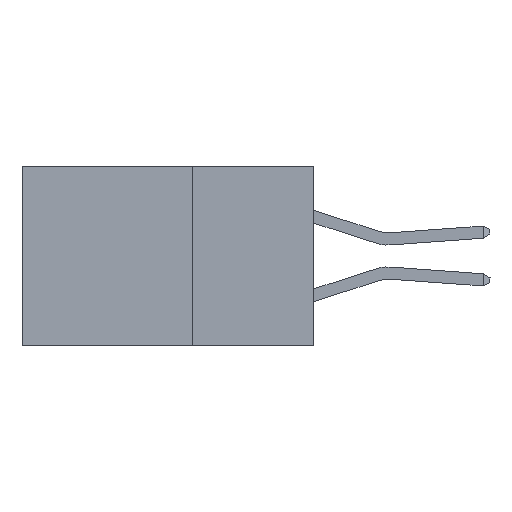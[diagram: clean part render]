
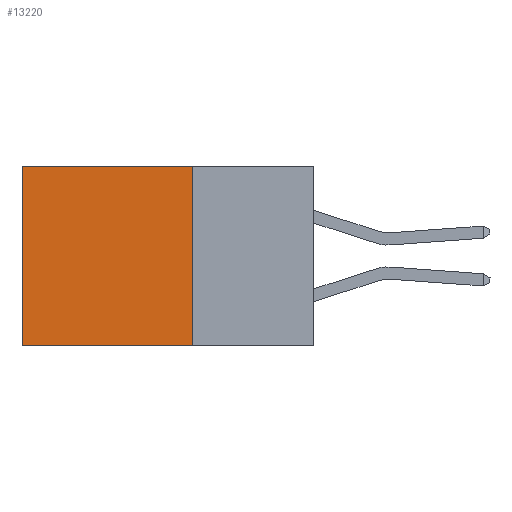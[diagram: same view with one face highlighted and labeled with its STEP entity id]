
A CAD part, left-side view. The second image highlights one B-rep face of the part: STEP entity #13220.
In plain terms, the highlighted planar face has unit normal (-1, 0, 0).
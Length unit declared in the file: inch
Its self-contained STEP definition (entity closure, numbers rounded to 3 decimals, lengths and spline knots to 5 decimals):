
#343 = VECTOR ( 'NONE', #6720, 39.37008 ) ;
#418 = CARTESIAN_POINT ( 'NONE',  ( 0.2875, 0.25, -0.37 ) ) ;
#1575 = CARTESIAN_POINT ( 'NONE',  ( 0.2875, 0.6, 0. ) ) ;
#3010 = VERTEX_POINT ( 'NONE', #418 ) ;
#3267 = PLANE ( 'NONE',  #4770 ) ;
#3728 = LINE ( 'NONE', #4398, #9536 ) ;
#3859 = VERTEX_POINT ( 'NONE', #1575 ) ;
#4029 = EDGE_CURVE ( 'NONE', #4447, #3010, #9342, .T. ) ;
#4398 = CARTESIAN_POINT ( 'NONE',  ( 0.2875, 0.25, -0.37 ) ) ;
#4447 = VERTEX_POINT ( 'NONE', #6505 ) ;
#4452 = DIRECTION ( 'NONE',  ( 0., 1., 0. ) ) ;
#4518 = DIRECTION ( 'NONE',  ( 1., 0., 0. ) ) ;
#4770 = AXIS2_PLACEMENT_3D ( 'NONE', #10228, #4518, #12395 ) ;
#4926 = ORIENTED_EDGE ( 'NONE', *, *, #6169, .T. ) ;
#5045 = FACE_OUTER_BOUND ( 'NONE', #13410, .T. ) ;
#5629 = EDGE_CURVE ( 'NONE', #3859, #12016, #14111, .T. ) ;
#5664 = VECTOR ( 'NONE', #6521, 39.37008 ) ;
#6169 = EDGE_CURVE ( 'NONE', #4447, #3859, #7441, .T. ) ;
#6384 = EDGE_CURVE ( 'NONE', #3010, #12016, #3728, .T. ) ;
#6505 = CARTESIAN_POINT ( 'NONE',  ( 0.2875, 0.25, 0. ) ) ;
#6521 = DIRECTION ( 'NONE',  ( 0., 0., -1. ) ) ;
#6720 = DIRECTION ( 'NONE',  ( 0., 0., -1. ) ) ;
#6965 = ORIENTED_EDGE ( 'NONE', *, *, #4029, .F. ) ;
#7441 = LINE ( 'NONE', #8635, #13586 ) ;
#8635 = CARTESIAN_POINT ( 'NONE',  ( 0.2875, 0.25, 0. ) ) ;
#9342 = LINE ( 'NONE', #10117, #343 ) ;
#9536 = VECTOR ( 'NONE', #4452, 39.37008 ) ;
#9586 = ORIENTED_EDGE ( 'NONE', *, *, #5629, .T. ) ;
#10117 = CARTESIAN_POINT ( 'NONE',  ( 0.2875, 0.25, 0. ) ) ;
#10228 = CARTESIAN_POINT ( 'NONE',  ( 0.2875, 0.25, 0. ) ) ;
#10572 = CARTESIAN_POINT ( 'NONE',  ( 0.2875, 0.6, -0.37 ) ) ;
#12016 = VERTEX_POINT ( 'NONE', #10572 ) ;
#12395 = DIRECTION ( 'NONE',  ( 0., 0., -1. ) ) ;
#13098 = CARTESIAN_POINT ( 'NONE',  ( 0.2875, 0.6, 0. ) ) ;
#13220 = ADVANCED_FACE ( 'NONE', ( #5045 ), #3267, .F. ) ;
#13410 = EDGE_LOOP ( 'NONE', ( #9586, #14274, #6965, #4926 ) ) ;
#13586 = VECTOR ( 'NONE', #13997, 39.37008 ) ;
#13997 = DIRECTION ( 'NONE',  ( 0., 1., 0. ) ) ;
#14111 = LINE ( 'NONE', #13098, #5664 ) ;
#14274 = ORIENTED_EDGE ( 'NONE', *, *, #6384, .F. ) ;
